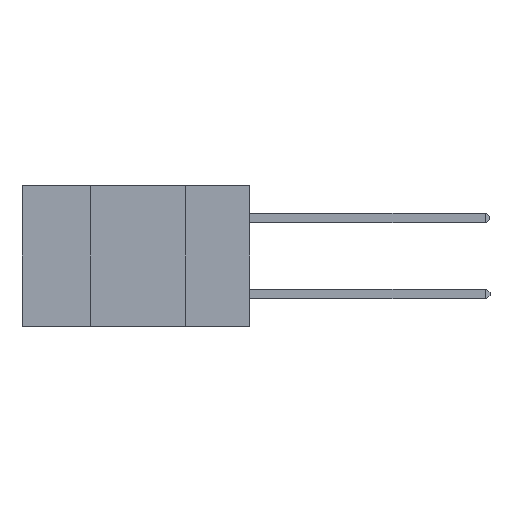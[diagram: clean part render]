
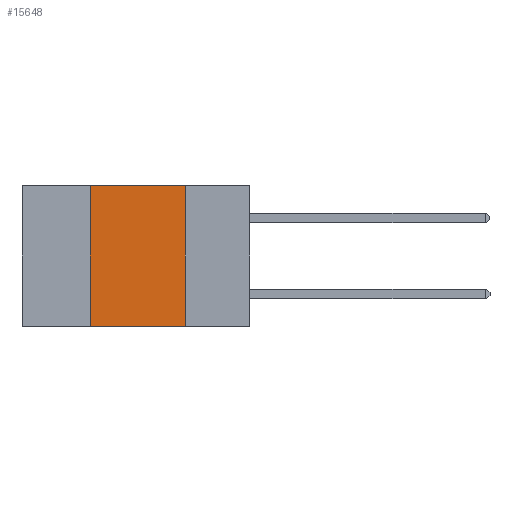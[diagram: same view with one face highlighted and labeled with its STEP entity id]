
A CAD part, left-side view. The second image highlights one B-rep face of the part: STEP entity #15648.
In plain terms, the highlighted planar face has unit normal (-1, 0, 0).
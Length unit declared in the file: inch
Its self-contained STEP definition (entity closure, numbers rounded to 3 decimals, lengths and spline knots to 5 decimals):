
#852 = AXIS2_PLACEMENT_3D ( 'NONE', #14146, #19463, #17731 ) ;
#860 = EDGE_CURVE ( 'NONE', #17831, #13788, #12172, .T. ) ;
#2378 = CARTESIAN_POINT ( 'NONE',  ( 0., 0.17, 0. ) ) ;
#3793 = DIRECTION ( 'NONE',  ( 0., -1., 0. ) ) ;
#3925 = EDGE_CURVE ( 'NONE', #13788, #9483, #10239, .T. ) ;
#6059 = VECTOR ( 'NONE', #6635, 39.37008 ) ;
#6273 = EDGE_CURVE ( 'NONE', #11832, #17831, #10984, .T. ) ;
#6635 = DIRECTION ( 'NONE',  ( 0., 0., 1. ) ) ;
#7523 = CARTESIAN_POINT ( 'NONE',  ( 0., 0.6, -0.37 ) ) ;
#8936 = VECTOR ( 'NONE', #3793, 39.37008 ) ;
#9483 = VERTEX_POINT ( 'NONE', #11965 ) ;
#9897 = CARTESIAN_POINT ( 'NONE',  ( 0., 0.42, -0.37 ) ) ;
#10239 = LINE ( 'NONE', #2378, #19896 ) ;
#10325 = ORIENTED_EDGE ( 'NONE', *, *, #3925, .F. ) ;
#10984 = LINE ( 'NONE', #13977, #6059 ) ;
#11832 = VERTEX_POINT ( 'NONE', #9897 ) ;
#11965 = CARTESIAN_POINT ( 'NONE',  ( 0., 0.17, -0.37 ) ) ;
#12172 = LINE ( 'NONE', #12749, #15865 ) ;
#12436 = DIRECTION ( 'NONE',  ( 0., -1., 0. ) ) ;
#12749 = CARTESIAN_POINT ( 'NONE',  ( 0., 0.6, 0. ) ) ;
#13788 = VERTEX_POINT ( 'NONE', #13985 ) ;
#13977 = CARTESIAN_POINT ( 'NONE',  ( 0., 0.42, 0. ) ) ;
#13985 = CARTESIAN_POINT ( 'NONE',  ( 0., 0.17, 0. ) ) ;
#14146 = CARTESIAN_POINT ( 'NONE',  ( 0., 0.6, 0. ) ) ;
#14392 = ORIENTED_EDGE ( 'NONE', *, *, #6273, .F. ) ;
#14986 = LINE ( 'NONE', #7523, #8936 ) ;
#15418 = DIRECTION ( 'NONE',  ( 0., 0., -1. ) ) ;
#15648 = ADVANCED_FACE ( 'NONE', ( #22830 ), #15955, .F. ) ;
#15865 = VECTOR ( 'NONE', #12436, 39.37008 ) ;
#15955 = PLANE ( 'NONE',  #852 ) ;
#16874 = EDGE_CURVE ( 'NONE', #11832, #9483, #14986, .T. ) ;
#17370 = CARTESIAN_POINT ( 'NONE',  ( 0., 0.42, 0. ) ) ;
#17731 = DIRECTION ( 'NONE',  ( 0., 0., -1. ) ) ;
#17831 = VERTEX_POINT ( 'NONE', #17370 ) ;
#19463 = DIRECTION ( 'NONE',  ( 1., 0., 0. ) ) ;
#19896 = VECTOR ( 'NONE', #15418, 39.37008 ) ;
#20815 = ORIENTED_EDGE ( 'NONE', *, *, #16874, .T. ) ;
#21663 = ORIENTED_EDGE ( 'NONE', *, *, #860, .F. ) ;
#22830 = FACE_OUTER_BOUND ( 'NONE', #23422, .T. ) ;
#23422 = EDGE_LOOP ( 'NONE', ( #10325, #21663, #14392, #20815 ) ) ;
